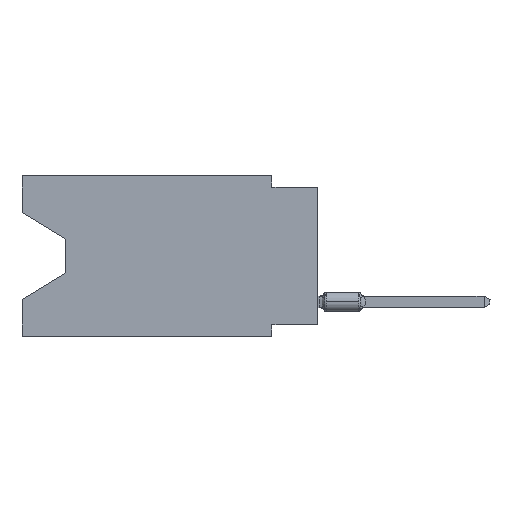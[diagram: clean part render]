
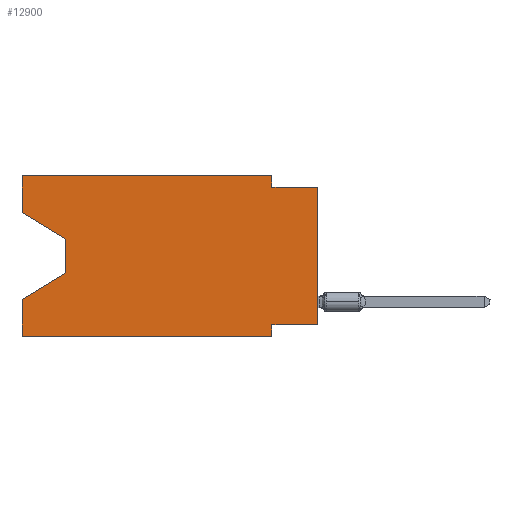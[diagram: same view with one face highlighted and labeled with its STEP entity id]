
A CAD part, left-side view. The second image highlights one B-rep face of the part: STEP entity #12900.
In plain terms, the highlighted planar face has unit normal (-1, 0, 0).
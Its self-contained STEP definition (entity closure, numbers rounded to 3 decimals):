
#186 = VERTEX_POINT ( 'NONE', #32377 ) ;
#290 = DIRECTION ( 'NONE',  ( 0., 0., -1. ) ) ;
#483 = CARTESIAN_POINT ( 'NONE',  ( 0., 0., -8.255 ) ) ;
#584 = CARTESIAN_POINT ( 'NONE',  ( 0., 16.383, 0. ) ) ;
#1952 = LINE ( 'NONE', #15836, #3951 ) ;
#2497 = EDGE_CURVE ( 'NONE', #12515, #22066, #13648, .T. ) ;
#2550 = DIRECTION ( 'NONE',  ( 0., 0., -1. ) ) ;
#2558 = ORIENTED_EDGE ( 'NONE', *, *, #2775, .T. ) ;
#2775 = EDGE_CURVE ( 'NONE', #31697, #3574, #3780, .T. ) ;
#2803 = ORIENTED_EDGE ( 'NONE', *, *, #6798, .T. ) ;
#2935 = CARTESIAN_POINT ( 'NONE',  ( 0., 13.97, -5.385 ) ) ;
#3062 = ORIENTED_EDGE ( 'NONE', *, *, #28950, .F. ) ;
#3362 = VECTOR ( 'NONE', #290, 1000. ) ;
#3574 = VERTEX_POINT ( 'NONE', #9644 ) ;
#3679 = FACE_OUTER_BOUND ( 'NONE', #5673, .T. ) ;
#3720 = CARTESIAN_POINT ( 'NONE',  ( 0., 2.54, -0.635 ) ) ;
#3780 = LINE ( 'NONE', #9256, #29253 ) ;
#3938 = LINE ( 'NONE', #17646, #7985 ) ;
#3951 = VECTOR ( 'NONE', #21829, 1000. ) ;
#4583 = DIRECTION ( 'NONE',  ( 0., -1., 0. ) ) ;
#5031 = EDGE_CURVE ( 'NONE', #3574, #12060, #13497, .T. ) ;
#5547 = VERTEX_POINT ( 'NONE', #16717 ) ;
#5648 = DIRECTION ( 'NONE',  ( 0., 1., 0. ) ) ;
#5673 = EDGE_LOOP ( 'NONE', ( #2558, #11261, #2803, #32119, #35226, #9420, #7990, #21268, #23617, #35618, #3062, #15620 ) ) ;
#6551 = VERTEX_POINT ( 'NONE', #34143 ) ;
#6711 = VECTOR ( 'NONE', #35600, 1000. ) ;
#6798 = EDGE_CURVE ( 'NONE', #12060, #32338, #24649, .T. ) ;
#7985 = VECTOR ( 'NONE', #31315, 1000. ) ;
#7990 = ORIENTED_EDGE ( 'NONE', *, *, #13156, .F. ) ;
#8296 = VECTOR ( 'NONE', #2550, 1000. ) ;
#8629 = CARTESIAN_POINT ( 'NONE',  ( 0., 0., 0. ) ) ;
#9140 = DIRECTION ( 'NONE',  ( 1., 0., 0. ) ) ;
#9256 = CARTESIAN_POINT ( 'NONE',  ( 0., 16.383, -2.038 ) ) ;
#9374 = DIRECTION ( 'NONE',  ( 0., 0., 1. ) ) ;
#9420 = ORIENTED_EDGE ( 'NONE', *, *, #18596, .F. ) ;
#9644 = CARTESIAN_POINT ( 'NONE',  ( 0., 13.97, -3.505 ) ) ;
#11261 = ORIENTED_EDGE ( 'NONE', *, *, #5031, .T. ) ;
#11509 = VERTEX_POINT ( 'NONE', #28994 ) ;
#11879 = DIRECTION ( 'NONE',  ( 0., -1., 0. ) ) ;
#12060 = VERTEX_POINT ( 'NONE', #22751 ) ;
#12515 = VERTEX_POINT ( 'NONE', #3720 ) ;
#12900 = ADVANCED_FACE ( 'NONE', ( #3679 ), #23371, .F. ) ;
#12959 = EDGE_CURVE ( 'NONE', #186, #11509, #19726, .T. ) ;
#13156 = EDGE_CURVE ( 'NONE', #30972, #5547, #35764, .T. ) ;
#13497 = LINE ( 'NONE', #24235, #8296 ) ;
#13648 = LINE ( 'NONE', #35539, #15858 ) ;
#14439 = DIRECTION ( 'NONE',  ( 0., 0., -1. ) ) ;
#14646 = EDGE_CURVE ( 'NONE', #31697, #27700, #3938, .T. ) ;
#14799 = CARTESIAN_POINT ( 'NONE',  ( 0., 16.383, -8.89 ) ) ;
#15525 = LINE ( 'NONE', #20642, #16104 ) ;
#15620 = ORIENTED_EDGE ( 'NONE', *, *, #14646, .F. ) ;
#15762 = EDGE_CURVE ( 'NONE', #186, #32338, #25964, .T. ) ;
#15836 = CARTESIAN_POINT ( 'NONE',  ( 0., 2.54, 0. ) ) ;
#15858 = VECTOR ( 'NONE', #16393, 1000. ) ;
#16104 = VECTOR ( 'NONE', #4583, 1000. ) ;
#16208 = AXIS2_PLACEMENT_3D ( 'NONE', #584, #9140, #14439 ) ;
#16393 = DIRECTION ( 'NONE',  ( 0., -1., 0. ) ) ;
#16717 = CARTESIAN_POINT ( 'NONE',  ( 0., 2.54, -8.255 ) ) ;
#16801 = VECTOR ( 'NONE', #27798, 1000. ) ;
#17646 = CARTESIAN_POINT ( 'NONE',  ( 0., 16.383, 0. ) ) ;
#18596 = EDGE_CURVE ( 'NONE', #5547, #11509, #25829, .T. ) ;
#19726 = LINE ( 'NONE', #14799, #30811 ) ;
#20642 = CARTESIAN_POINT ( 'NONE',  ( 0., 16.383, 0. ) ) ;
#20643 = CARTESIAN_POINT ( 'NONE',  ( 0., 0., -0.635 ) ) ;
#20944 = VECTOR ( 'NONE', #5648, 1000. ) ;
#21268 = ORIENTED_EDGE ( 'NONE', *, *, #23558, .T. ) ;
#21829 = DIRECTION ( 'NONE',  ( 0., 0., -1. ) ) ;
#22066 = VERTEX_POINT ( 'NONE', #20643 ) ;
#22751 = CARTESIAN_POINT ( 'NONE',  ( 0., 13.97, -5.385 ) ) ;
#22958 = EDGE_CURVE ( 'NONE', #6551, #12515, #1952, .T. ) ;
#23371 = PLANE ( 'NONE',  #16208 ) ;
#23558 = EDGE_CURVE ( 'NONE', #30972, #22066, #33624, .T. ) ;
#23617 = ORIENTED_EDGE ( 'NONE', *, *, #2497, .F. ) ;
#24235 = CARTESIAN_POINT ( 'NONE',  ( 0., 13.97, -3.505 ) ) ;
#24649 = LINE ( 'NONE', #2935, #6711 ) ;
#25829 = LINE ( 'NONE', #28029, #3362 ) ;
#25964 = LINE ( 'NONE', #34367, #28945 ) ;
#27700 = VERTEX_POINT ( 'NONE', #28694 ) ;
#27798 = DIRECTION ( 'NONE',  ( 0., 0., 1. ) ) ;
#28029 = CARTESIAN_POINT ( 'NONE',  ( 0., 2.54, -8.89 ) ) ;
#28694 = CARTESIAN_POINT ( 'NONE',  ( 0., 16.383, 0. ) ) ;
#28945 = VECTOR ( 'NONE', #9374, 1000. ) ;
#28950 = EDGE_CURVE ( 'NONE', #27700, #6551, #15525, .T. ) ;
#28994 = CARTESIAN_POINT ( 'NONE',  ( 0., 2.54, -8.89 ) ) ;
#29253 = VECTOR ( 'NONE', #33907, 1000. ) ;
#30811 = VECTOR ( 'NONE', #11879, 1000. ) ;
#30972 = VERTEX_POINT ( 'NONE', #483 ) ;
#31011 = CARTESIAN_POINT ( 'NONE',  ( 0., 16.383, -2.038 ) ) ;
#31315 = DIRECTION ( 'NONE',  ( 0., 0., 1. ) ) ;
#31697 = VERTEX_POINT ( 'NONE', #31011 ) ;
#32119 = ORIENTED_EDGE ( 'NONE', *, *, #15762, .F. ) ;
#32338 = VERTEX_POINT ( 'NONE', #35843 ) ;
#32377 = CARTESIAN_POINT ( 'NONE',  ( 0., 16.383, -8.89 ) ) ;
#33029 = CARTESIAN_POINT ( 'NONE',  ( 0., 0., -8.255 ) ) ;
#33624 = LINE ( 'NONE', #8629, #16801 ) ;
#33907 = DIRECTION ( 'NONE',  ( 0., -0.855, -0.519 ) ) ;
#34143 = CARTESIAN_POINT ( 'NONE',  ( 0., 2.54, 0. ) ) ;
#34367 = CARTESIAN_POINT ( 'NONE',  ( 0., 16.383, 0. ) ) ;
#35226 = ORIENTED_EDGE ( 'NONE', *, *, #12959, .T. ) ;
#35539 = CARTESIAN_POINT ( 'NONE',  ( 0., 0., -0.635 ) ) ;
#35600 = DIRECTION ( 'NONE',  ( 0., 0.855, -0.519 ) ) ;
#35618 = ORIENTED_EDGE ( 'NONE', *, *, #22958, .F. ) ;
#35764 = LINE ( 'NONE', #33029, #20944 ) ;
#35843 = CARTESIAN_POINT ( 'NONE',  ( 0., 16.383, -6.852 ) ) ;
